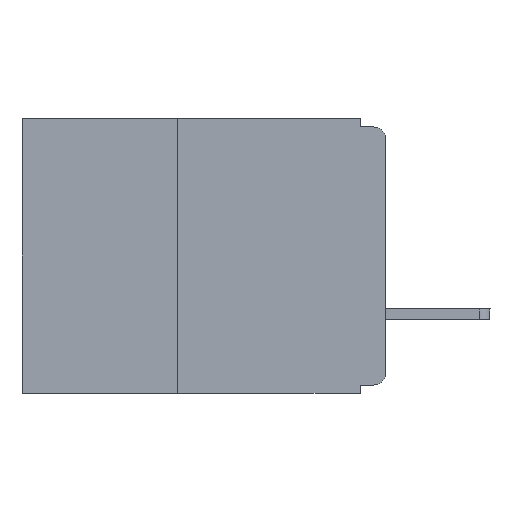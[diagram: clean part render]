
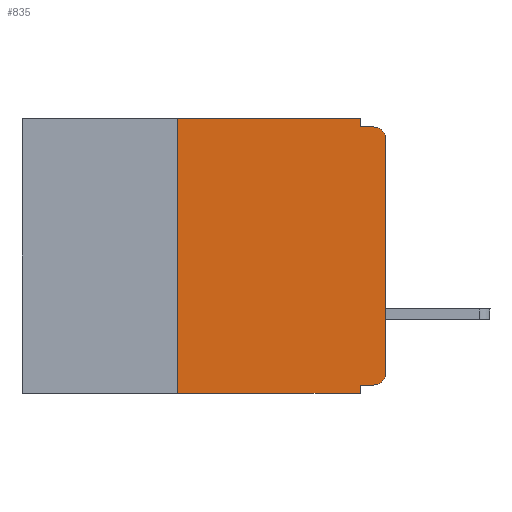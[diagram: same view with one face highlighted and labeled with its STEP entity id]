
A CAD part, left-side view. The second image highlights one B-rep face of the part: STEP entity #835.
In plain terms, the highlighted planar face has unit normal (-1, 0, 0).
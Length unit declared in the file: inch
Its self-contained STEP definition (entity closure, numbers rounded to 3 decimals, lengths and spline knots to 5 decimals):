
#132 = LINE ( 'NONE', #9759, #14000 ) ;
#134 = VERTEX_POINT ( 'NONE', #4138 ) ;
#143 = DIRECTION ( 'NONE',  ( -1., 0., 0. ) ) ;
#180 = AXIS2_PLACEMENT_3D ( 'NONE', #6460, #15030, #7959 ) ;
#394 = CIRCLE ( 'NONE', #1317, 0.015 ) ;
#606 = ORIENTED_EDGE ( 'NONE', *, *, #2404, .F. ) ;
#754 = VECTOR ( 'NONE', #844, 39.37008 ) ;
#807 = EDGE_CURVE ( 'NONE', #5710, #11872, #4190, .T. ) ;
#835 = ADVANCED_FACE ( 'NONE', ( #6879 ), #11495, .F. ) ;
#844 = DIRECTION ( 'NONE',  ( 0., -1., 0. ) ) ;
#855 = CARTESIAN_POINT ( 'NONE',  ( 0., 0.031, 0. ) ) ;
#1317 = AXIS2_PLACEMENT_3D ( 'NONE', #3497, #143, #8207 ) ;
#1521 = ORIENTED_EDGE ( 'NONE', *, *, #1831, .F. ) ;
#1593 = CARTESIAN_POINT ( 'NONE',  ( 0., 0.25, -0.33 ) ) ;
#1682 = CARTESIAN_POINT ( 'NONE',  ( 0., 0., -0.32 ) ) ;
#1728 = DIRECTION ( 'NONE',  ( 0., 1., 0. ) ) ;
#1831 = EDGE_CURVE ( 'NONE', #13127, #134, #10834, .T. ) ;
#1940 = DIRECTION ( 'NONE',  ( 0., -1., 0. ) ) ;
#2087 = DIRECTION ( 'NONE',  ( 1., 0., 0. ) ) ;
#2372 = CARTESIAN_POINT ( 'NONE',  ( 0., 0.031, 0. ) ) ;
#2404 = EDGE_CURVE ( 'NONE', #13424, #10657, #13063, .T. ) ;
#2429 = LINE ( 'NONE', #3358, #10383 ) ;
#2786 = ORIENTED_EDGE ( 'NONE', *, *, #6168, .F. ) ;
#2992 = DIRECTION ( 'NONE',  ( 0., 0., 1. ) ) ;
#3180 = CARTESIAN_POINT ( 'NONE',  ( 0., 0., -0.01 ) ) ;
#3280 = EDGE_CURVE ( 'NONE', #8792, #13424, #9763, .T. ) ;
#3358 = CARTESIAN_POINT ( 'NONE',  ( 0., 0., 0. ) ) ;
#3497 = CARTESIAN_POINT ( 'NONE',  ( 0., 0.015, -0.305 ) ) ;
#3637 = VECTOR ( 'NONE', #1940, 39.37008 ) ;
#3877 = LINE ( 'NONE', #1593, #12940 ) ;
#3918 = CARTESIAN_POINT ( 'NONE',  ( 0., 0.031, -0.33 ) ) ;
#4138 = CARTESIAN_POINT ( 'NONE',  ( 0., 0.031, -0.01 ) ) ;
#4190 = CIRCLE ( 'NONE', #180, 0.015 ) ;
#4665 = VERTEX_POINT ( 'NONE', #7028 ) ;
#4673 = ORIENTED_EDGE ( 'NONE', *, *, #3280, .F. ) ;
#5087 = ORIENTED_EDGE ( 'NONE', *, *, #11660, .T. ) ;
#5592 = EDGE_CURVE ( 'NONE', #9848, #4665, #3877, .T. ) ;
#5629 = CARTESIAN_POINT ( 'NONE',  ( 0., 0.031, -0.33 ) ) ;
#5668 = EDGE_CURVE ( 'NONE', #6943, #5710, #2429, .T. ) ;
#5680 = CARTESIAN_POINT ( 'NONE',  ( 0., 0.437, -0.33 ) ) ;
#5710 = VERTEX_POINT ( 'NONE', #11593 ) ;
#6168 = EDGE_CURVE ( 'NONE', #4665, #13127, #132, .T. ) ;
#6460 = CARTESIAN_POINT ( 'NONE',  ( 0., 0.015, -0.025 ) ) ;
#6879 = FACE_OUTER_BOUND ( 'NONE', #14006, .T. ) ;
#6943 = VERTEX_POINT ( 'NONE', #11168 ) ;
#7028 = CARTESIAN_POINT ( 'NONE',  ( 0., 0.25, 0. ) ) ;
#7764 = ORIENTED_EDGE ( 'NONE', *, *, #13376, .F. ) ;
#7959 = DIRECTION ( 'NONE',  ( 0., 0., -1. ) ) ;
#8207 = DIRECTION ( 'NONE',  ( 0., 0., -1. ) ) ;
#8792 = VERTEX_POINT ( 'NONE', #11569 ) ;
#9244 = CARTESIAN_POINT ( 'NONE',  ( 0., 0.437, 0. ) ) ;
#9759 = CARTESIAN_POINT ( 'NONE',  ( 0., 0.437, 0. ) ) ;
#9763 = LINE ( 'NONE', #1682, #13984 ) ;
#9812 = ORIENTED_EDGE ( 'NONE', *, *, #807, .T. ) ;
#9825 = ORIENTED_EDGE ( 'NONE', *, *, #11503, .T. ) ;
#9848 = VERTEX_POINT ( 'NONE', #10605 ) ;
#10087 = DIRECTION ( 'NONE',  ( 0., 0., -1. ) ) ;
#10193 = DIRECTION ( 'NONE',  ( 0., 0., -1. ) ) ;
#10383 = VECTOR ( 'NONE', #13880, 39.37008 ) ;
#10605 = CARTESIAN_POINT ( 'NONE',  ( 0., 0.25, -0.33 ) ) ;
#10657 = VERTEX_POINT ( 'NONE', #5629 ) ;
#10683 = LINE ( 'NONE', #3180, #3637 ) ;
#10834 = LINE ( 'NONE', #855, #11767 ) ;
#11168 = CARTESIAN_POINT ( 'NONE',  ( 0., 0., -0.305 ) ) ;
#11299 = CARTESIAN_POINT ( 'NONE',  ( 0., 0.031, -0.32 ) ) ;
#11495 = PLANE ( 'NONE',  #14373 ) ;
#11503 = EDGE_CURVE ( 'NONE', #8792, #6943, #394, .T. ) ;
#11569 = CARTESIAN_POINT ( 'NONE',  ( 0., 0.015, -0.32 ) ) ;
#11593 = CARTESIAN_POINT ( 'NONE',  ( 0., 0., -0.025 ) ) ;
#11660 = EDGE_CURVE ( 'NONE', #9848, #10657, #14430, .T. ) ;
#11767 = VECTOR ( 'NONE', #10087, 39.37008 ) ;
#11872 = VERTEX_POINT ( 'NONE', #14347 ) ;
#12095 = DIRECTION ( 'NONE',  ( 0., -1., 0. ) ) ;
#12433 = ORIENTED_EDGE ( 'NONE', *, *, #5668, .T. ) ;
#12600 = ORIENTED_EDGE ( 'NONE', *, *, #5592, .F. ) ;
#12940 = VECTOR ( 'NONE', #2992, 39.37008 ) ;
#13063 = LINE ( 'NONE', #3918, #15119 ) ;
#13127 = VERTEX_POINT ( 'NONE', #2372 ) ;
#13376 = EDGE_CURVE ( 'NONE', #134, #11872, #10683, .T. ) ;
#13424 = VERTEX_POINT ( 'NONE', #11299 ) ;
#13880 = DIRECTION ( 'NONE',  ( 0., 0., 1. ) ) ;
#13984 = VECTOR ( 'NONE', #1728, 39.37008 ) ;
#14000 = VECTOR ( 'NONE', #12095, 39.37008 ) ;
#14006 = EDGE_LOOP ( 'NONE', ( #12433, #9812, #7764, #1521, #2786, #12600, #5087, #606, #4673, #9825 ) ) ;
#14257 = DIRECTION ( 'NONE',  ( 0., 0., -1. ) ) ;
#14347 = CARTESIAN_POINT ( 'NONE',  ( 0., 0.015, -0.01 ) ) ;
#14373 = AXIS2_PLACEMENT_3D ( 'NONE', #9244, #2087, #10193 ) ;
#14430 = LINE ( 'NONE', #5680, #754 ) ;
#15030 = DIRECTION ( 'NONE',  ( -1., 0., 0. ) ) ;
#15119 = VECTOR ( 'NONE', #14257, 39.37008 ) ;
